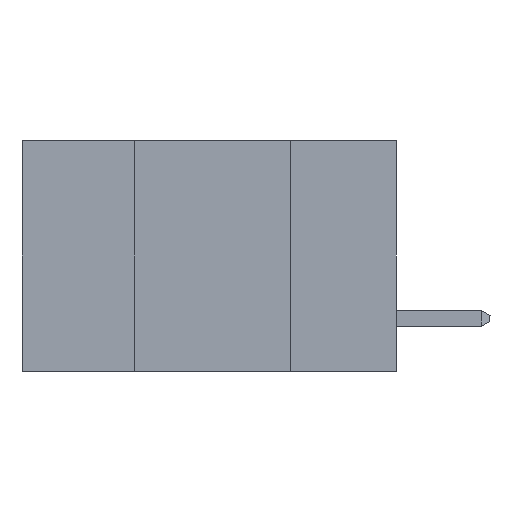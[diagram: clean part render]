
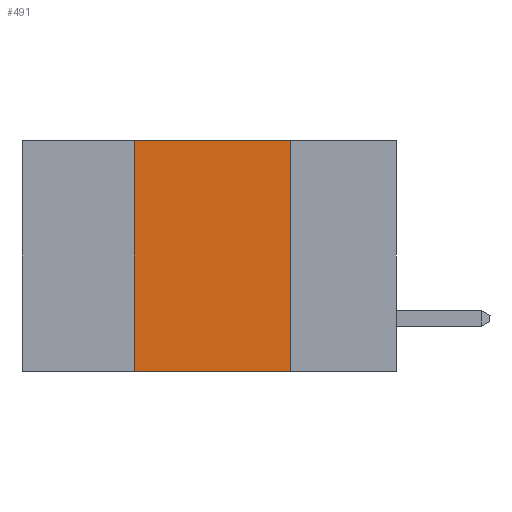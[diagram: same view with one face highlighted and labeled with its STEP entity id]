
A CAD part, left-side view. The second image highlights one B-rep face of the part: STEP entity #491.
In plain terms, the highlighted planar face has unit normal (-1, 0, 0).
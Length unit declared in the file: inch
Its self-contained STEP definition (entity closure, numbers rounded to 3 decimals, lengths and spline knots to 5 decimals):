
#491 = ADVANCED_FACE ( 'NONE', ( #10669 ), #2121, .F. ) ;
#951 = LINE ( 'NONE', #3512, #11341 ) ;
#1144 = CARTESIAN_POINT ( 'NONE',  ( 0., 0.42, -0.37 ) ) ;
#1468 = DIRECTION ( 'NONE',  ( 0., -1., 0. ) ) ;
#2121 = PLANE ( 'NONE',  #14112 ) ;
#2632 = LINE ( 'NONE', #2714, #4932 ) ;
#2714 = CARTESIAN_POINT ( 'NONE',  ( 0., 0.6, -0.37 ) ) ;
#3013 = VERTEX_POINT ( 'NONE', #14076 ) ;
#3385 = VERTEX_POINT ( 'NONE', #13317 ) ;
#3466 = DIRECTION ( 'NONE',  ( 0., -1., 0. ) ) ;
#3512 = CARTESIAN_POINT ( 'NONE',  ( 0., 0.42, -0.37 ) ) ;
#4374 = DIRECTION ( 'NONE',  ( 1., 0., 0. ) ) ;
#4652 = EDGE_CURVE ( 'NONE', #13012, #4678, #2632, .T. ) ;
#4678 = VERTEX_POINT ( 'NONE', #12671 ) ;
#4932 = VECTOR ( 'NONE', #1468, 39.37008 ) ;
#5688 = LINE ( 'NONE', #10267, #7938 ) ;
#6093 = DIRECTION ( 'NONE',  ( 0., 0., 1. ) ) ;
#6571 = EDGE_CURVE ( 'NONE', #3385, #4678, #5688, .T. ) ;
#6668 = EDGE_CURVE ( 'NONE', #13012, #3013, #951, .T. ) ;
#7554 = LINE ( 'NONE', #9693, #10157 ) ;
#7938 = VECTOR ( 'NONE', #15344, 39.37008 ) ;
#9344 = ORIENTED_EDGE ( 'NONE', *, *, #6668, .F. ) ;
#9693 = CARTESIAN_POINT ( 'NONE',  ( 0., 0.6, 0. ) ) ;
#10157 = VECTOR ( 'NONE', #3466, 39.37008 ) ;
#10267 = CARTESIAN_POINT ( 'NONE',  ( 0., 0.17, -0.37 ) ) ;
#10669 = FACE_OUTER_BOUND ( 'NONE', #13926, .T. ) ;
#10924 = CARTESIAN_POINT ( 'NONE',  ( 0., 0.6, 0. ) ) ;
#11341 = VECTOR ( 'NONE', #6093, 39.37008 ) ;
#11881 = ORIENTED_EDGE ( 'NONE', *, *, #14324, .F. ) ;
#12666 = ORIENTED_EDGE ( 'NONE', *, *, #6571, .F. ) ;
#12671 = CARTESIAN_POINT ( 'NONE',  ( 0., 0.17, -0.37 ) ) ;
#13012 = VERTEX_POINT ( 'NONE', #1144 ) ;
#13317 = CARTESIAN_POINT ( 'NONE',  ( 0., 0.17, 0. ) ) ;
#13758 = ORIENTED_EDGE ( 'NONE', *, *, #4652, .T. ) ;
#13926 = EDGE_LOOP ( 'NONE', ( #12666, #11881, #9344, #13758 ) ) ;
#14076 = CARTESIAN_POINT ( 'NONE',  ( 0., 0.42, 0. ) ) ;
#14112 = AXIS2_PLACEMENT_3D ( 'NONE', #10924, #4374, #16000 ) ;
#14324 = EDGE_CURVE ( 'NONE', #3013, #3385, #7554, .T. ) ;
#15344 = DIRECTION ( 'NONE',  ( 0., 0., -1. ) ) ;
#16000 = DIRECTION ( 'NONE',  ( 0., 0., -1. ) ) ;
